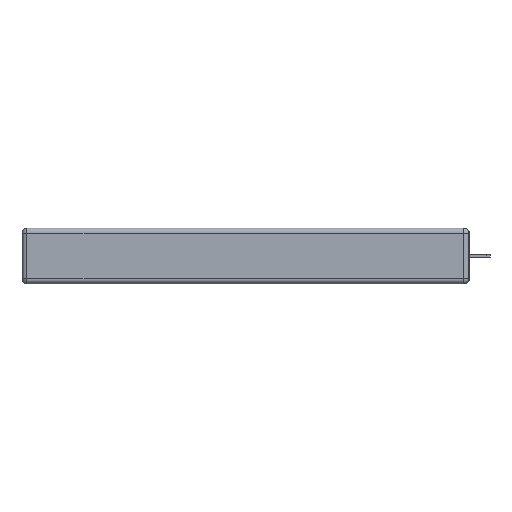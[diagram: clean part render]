
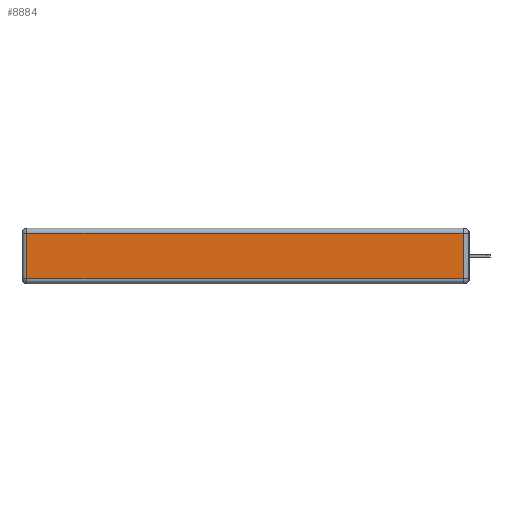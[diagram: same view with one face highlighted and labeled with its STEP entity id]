
A CAD part, left-side view. The second image highlights one B-rep face of the part: STEP entity #8884.
In plain terms, the highlighted planar face has unit normal (-1, 0, 0).
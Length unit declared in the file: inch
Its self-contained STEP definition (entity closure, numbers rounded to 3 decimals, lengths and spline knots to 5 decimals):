
#599 = VECTOR ( 'NONE', #5494, 39.37008 ) ;
#680 = VERTEX_POINT ( 'NONE', #12943 ) ;
#687 = DIRECTION ( 'NONE',  ( 0., 0., 1. ) ) ;
#1328 = EDGE_LOOP ( 'NONE', ( #4780, #4811, #3337, #6197 ) ) ;
#1712 = LINE ( 'NONE', #11199, #9089 ) ;
#2499 = VERTEX_POINT ( 'NONE', #6249 ) ;
#2551 = EDGE_CURVE ( 'NONE', #11380, #680, #8368, .T. ) ;
#2662 = DIRECTION ( 'NONE',  ( 0., 1., 0. ) ) ;
#3071 = CARTESIAN_POINT ( 'NONE',  ( 0., 2.72, -0.343 ) ) ;
#3337 = ORIENTED_EDGE ( 'NONE', *, *, #2551, .T. ) ;
#4622 = DIRECTION ( 'NONE',  ( -1., 0., 0. ) ) ;
#4752 = CARTESIAN_POINT ( 'NONE',  ( 0., 0.03, -0.03 ) ) ;
#4780 = ORIENTED_EDGE ( 'NONE', *, *, #14085, .T. ) ;
#4811 = ORIENTED_EDGE ( 'NONE', *, *, #12759, .T. ) ;
#4929 = PLANE ( 'NONE',  #10030 ) ;
#5433 = LINE ( 'NONE', #10037, #8620 ) ;
#5494 = DIRECTION ( 'NONE',  ( 0., 0., -1. ) ) ;
#5933 = CARTESIAN_POINT ( 'NONE',  ( 0., 0., -0.343 ) ) ;
#6197 = ORIENTED_EDGE ( 'NONE', *, *, #9866, .T. ) ;
#6249 = CARTESIAN_POINT ( 'NONE',  ( 0., 0.03, -0.313 ) ) ;
#6617 = DIRECTION ( 'NONE',  ( 0., -1., 0. ) ) ;
#7231 = VECTOR ( 'NONE', #2662, 39.37008 ) ;
#8368 = LINE ( 'NONE', #14510, #7231 ) ;
#8429 = FACE_OUTER_BOUND ( 'NONE', #1328, .T. ) ;
#8620 = VECTOR ( 'NONE', #687, 39.37008 ) ;
#8884 = ADVANCED_FACE ( 'NONE', ( #8429 ), #4929, .T. ) ;
#9022 = VERTEX_POINT ( 'NONE', #12370 ) ;
#9089 = VECTOR ( 'NONE', #6617, 39.37008 ) ;
#9866 = EDGE_CURVE ( 'NONE', #680, #9022, #12479, .T. ) ;
#10030 = AXIS2_PLACEMENT_3D ( 'NONE', #5933, #4622, #13155 ) ;
#10037 = CARTESIAN_POINT ( 'NONE',  ( 0., 0.03, -0.343 ) ) ;
#11199 = CARTESIAN_POINT ( 'NONE',  ( 0., 0., -0.313 ) ) ;
#11380 = VERTEX_POINT ( 'NONE', #4752 ) ;
#12370 = CARTESIAN_POINT ( 'NONE',  ( 0., 2.72, -0.313 ) ) ;
#12479 = LINE ( 'NONE', #3071, #599 ) ;
#12759 = EDGE_CURVE ( 'NONE', #2499, #11380, #5433, .T. ) ;
#12943 = CARTESIAN_POINT ( 'NONE',  ( 0., 2.72, -0.03 ) ) ;
#13155 = DIRECTION ( 'NONE',  ( 0., 0., 1. ) ) ;
#14085 = EDGE_CURVE ( 'NONE', #9022, #2499, #1712, .T. ) ;
#14510 = CARTESIAN_POINT ( 'NONE',  ( 0., 2.75, -0.03 ) ) ;
